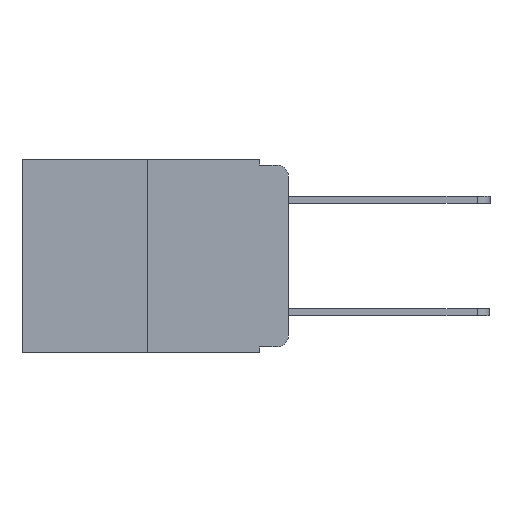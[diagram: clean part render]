
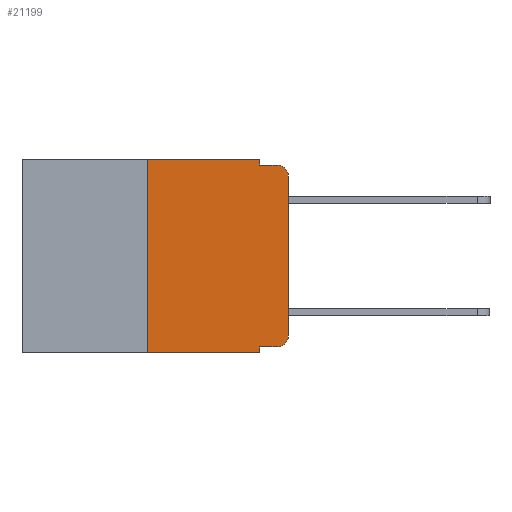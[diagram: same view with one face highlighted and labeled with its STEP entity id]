
A CAD part, left-side view. The second image highlights one B-rep face of the part: STEP entity #21199.
In plain terms, the highlighted planar face has unit normal (-1, 0, 0).
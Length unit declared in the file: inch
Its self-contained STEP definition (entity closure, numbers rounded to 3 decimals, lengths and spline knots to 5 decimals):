
#243 = CARTESIAN_POINT ( 'NONE',  ( 0., 0.051, 0. ) ) ;
#578 = DIRECTION ( 'NONE',  ( 0., 0., -1. ) ) ;
#651 = CARTESIAN_POINT ( 'NONE',  ( 0., 0., -0.313 ) ) ;
#773 = VERTEX_POINT ( 'NONE', #12010 ) ;
#1776 = LINE ( 'NONE', #14564, #12499 ) ;
#1891 = CARTESIAN_POINT ( 'NONE',  ( 0., 0.25, 0. ) ) ;
#2295 = EDGE_CURVE ( 'NONE', #7527, #16698, #15326, .T. ) ;
#2434 = CARTESIAN_POINT ( 'NONE',  ( 0., 0.473, -0.343 ) ) ;
#2829 = ORIENTED_EDGE ( 'NONE', *, *, #5612, .F. ) ;
#2859 = EDGE_CURVE ( 'NONE', #773, #7527, #9570, .T. ) ;
#3202 = CARTESIAN_POINT ( 'NONE',  ( 0., 0.051, -0.333 ) ) ;
#3795 = ORIENTED_EDGE ( 'NONE', *, *, #12726, .T. ) ;
#4178 = VECTOR ( 'NONE', #9241, 39.37008 ) ;
#4234 = CIRCLE ( 'NONE', #15428, 0.02 ) ;
#4317 = LINE ( 'NONE', #3202, #14252 ) ;
#4490 = VERTEX_POINT ( 'NONE', #6406 ) ;
#4596 = VERTEX_POINT ( 'NONE', #651 ) ;
#4759 = ORIENTED_EDGE ( 'NONE', *, *, #2295, .F. ) ;
#5218 = VECTOR ( 'NONE', #15526, 39.37008 ) ;
#5612 = EDGE_CURVE ( 'NONE', #20082, #4490, #1776, .T. ) ;
#5768 = CARTESIAN_POINT ( 'NONE',  ( 0., 0.02, -0.333 ) ) ;
#6053 = ORIENTED_EDGE ( 'NONE', *, *, #11333, .T. ) ;
#6140 = AXIS2_PLACEMENT_3D ( 'NONE', #10756, #12698, #578 ) ;
#6406 = CARTESIAN_POINT ( 'NONE',  ( 0., 0.02, -0.01 ) ) ;
#6485 = CIRCLE ( 'NONE', #20541, 0.02 ) ;
#6855 = VERTEX_POINT ( 'NONE', #19888 ) ;
#6894 = DIRECTION ( 'NONE',  ( 0., 0., 1. ) ) ;
#7332 = DIRECTION ( 'NONE',  ( 0., -1., 0. ) ) ;
#7527 = VERTEX_POINT ( 'NONE', #14138 ) ;
#7611 = CARTESIAN_POINT ( 'NONE',  ( 0., 0.051, -0.333 ) ) ;
#8617 = DIRECTION ( 'NONE',  ( 0., -1., 0. ) ) ;
#8752 = EDGE_CURVE ( 'NONE', #23821, #4490, #4234, .T. ) ;
#8801 = PLANE ( 'NONE',  #6140 ) ;
#8829 = EDGE_CURVE ( 'NONE', #9910, #4596, #6485, .T. ) ;
#8880 = LINE ( 'NONE', #16565, #17891 ) ;
#9241 = DIRECTION ( 'NONE',  ( 0., 0., 1. ) ) ;
#9570 = LINE ( 'NONE', #1891, #4178 ) ;
#9762 = DIRECTION ( 'NONE',  ( -1., 0., 0. ) ) ;
#9910 = VERTEX_POINT ( 'NONE', #5768 ) ;
#9919 = CARTESIAN_POINT ( 'NONE',  ( 0., 0.02, -0.313 ) ) ;
#10756 = CARTESIAN_POINT ( 'NONE',  ( 0., 0.473, 0. ) ) ;
#11333 = EDGE_CURVE ( 'NONE', #773, #6855, #16706, .T. ) ;
#11433 = LINE ( 'NONE', #24825, #15919 ) ;
#11626 = ORIENTED_EDGE ( 'NONE', *, *, #17372, .T. ) ;
#11886 = DIRECTION ( 'NONE',  ( 0., 0., -1. ) ) ;
#12010 = CARTESIAN_POINT ( 'NONE',  ( 0., 0.25, -0.343 ) ) ;
#12499 = VECTOR ( 'NONE', #16461, 39.37008 ) ;
#12698 = DIRECTION ( 'NONE',  ( 1., 0., 0. ) ) ;
#12712 = CARTESIAN_POINT ( 'NONE',  ( 0., 0.473, 0. ) ) ;
#12726 = EDGE_CURVE ( 'NONE', #13605, #9910, #4317, .T. ) ;
#13605 = VERTEX_POINT ( 'NONE', #7611 ) ;
#14138 = CARTESIAN_POINT ( 'NONE',  ( 0., 0.25, 0. ) ) ;
#14174 = CARTESIAN_POINT ( 'NONE',  ( 0., 0., -0.03 ) ) ;
#14252 = VECTOR ( 'NONE', #7332, 39.37008 ) ;
#14556 = EDGE_LOOP ( 'NONE', ( #11626, #22347, #2829, #19098, #4759, #15232, #6053, #22653, #3795, #24417 ) ) ;
#14564 = CARTESIAN_POINT ( 'NONE',  ( 0., 0.051, -0.01 ) ) ;
#14834 = EDGE_CURVE ( 'NONE', #16698, #20082, #20716, .T. ) ;
#15049 = EDGE_CURVE ( 'NONE', #13605, #6855, #11433, .T. ) ;
#15232 = ORIENTED_EDGE ( 'NONE', *, *, #2859, .F. ) ;
#15326 = LINE ( 'NONE', #12712, #24792 ) ;
#15428 = AXIS2_PLACEMENT_3D ( 'NONE', #21217, #9762, #23117 ) ;
#15526 = DIRECTION ( 'NONE',  ( 0., 0., -1. ) ) ;
#15919 = VECTOR ( 'NONE', #17394, 39.37008 ) ;
#16103 = VECTOR ( 'NONE', #8617, 39.37008 ) ;
#16461 = DIRECTION ( 'NONE',  ( 0., -1., 0. ) ) ;
#16565 = CARTESIAN_POINT ( 'NONE',  ( 0., 0., 0. ) ) ;
#16698 = VERTEX_POINT ( 'NONE', #243 ) ;
#16706 = LINE ( 'NONE', #2434, #16103 ) ;
#17372 = EDGE_CURVE ( 'NONE', #4596, #23821, #8880, .T. ) ;
#17394 = DIRECTION ( 'NONE',  ( 0., 0., -1. ) ) ;
#17421 = CARTESIAN_POINT ( 'NONE',  ( 0., 0.051, 0. ) ) ;
#17891 = VECTOR ( 'NONE', #6894, 39.37008 ) ;
#18329 = CARTESIAN_POINT ( 'NONE',  ( 0., 0.051, -0.01 ) ) ;
#18357 = DIRECTION ( 'NONE',  ( 0., -1., 0. ) ) ;
#19098 = ORIENTED_EDGE ( 'NONE', *, *, #14834, .F. ) ;
#19888 = CARTESIAN_POINT ( 'NONE',  ( 0., 0.051, -0.343 ) ) ;
#20082 = VERTEX_POINT ( 'NONE', #18329 ) ;
#20541 = AXIS2_PLACEMENT_3D ( 'NONE', #9919, #23280, #11886 ) ;
#20716 = LINE ( 'NONE', #17421, #5218 ) ;
#21199 = ADVANCED_FACE ( 'NONE', ( #24427 ), #8801, .F. ) ;
#21217 = CARTESIAN_POINT ( 'NONE',  ( 0., 0.02, -0.03 ) ) ;
#22347 = ORIENTED_EDGE ( 'NONE', *, *, #8752, .T. ) ;
#22653 = ORIENTED_EDGE ( 'NONE', *, *, #15049, .F. ) ;
#23117 = DIRECTION ( 'NONE',  ( 0., 0., -1. ) ) ;
#23280 = DIRECTION ( 'NONE',  ( -1., 0., 0. ) ) ;
#23821 = VERTEX_POINT ( 'NONE', #14174 ) ;
#24417 = ORIENTED_EDGE ( 'NONE', *, *, #8829, .T. ) ;
#24427 = FACE_OUTER_BOUND ( 'NONE', #14556, .T. ) ;
#24792 = VECTOR ( 'NONE', #18357, 39.37008 ) ;
#24825 = CARTESIAN_POINT ( 'NONE',  ( 0., 0.051, 0. ) ) ;
